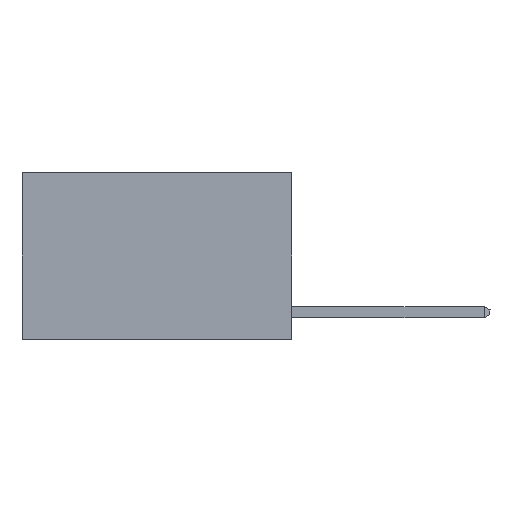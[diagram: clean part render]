
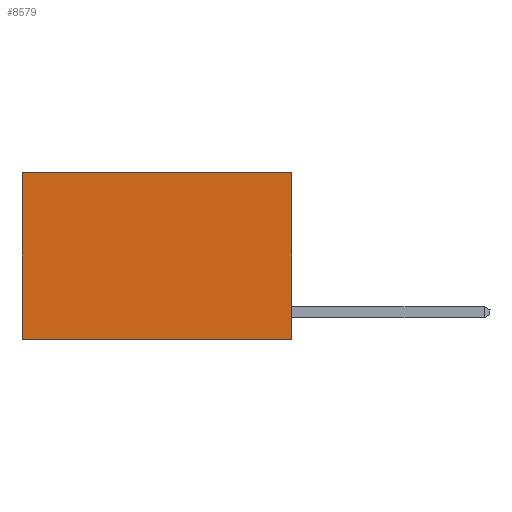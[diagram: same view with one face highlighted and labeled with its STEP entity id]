
A CAD part, left-side view. The second image highlights one B-rep face of the part: STEP entity #8579.
In plain terms, the highlighted planar face has unit normal (-1, 0, 0).
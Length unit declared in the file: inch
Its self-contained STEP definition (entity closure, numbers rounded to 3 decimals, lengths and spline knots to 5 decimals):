
#87 = DIRECTION ( 'NONE',  ( 0., 0., -1. ) ) ;
#495 = CARTESIAN_POINT ( 'NONE',  ( 0.2625, 0., 0. ) ) ;
#580 = VERTEX_POINT ( 'NONE', #14620 ) ;
#915 = VECTOR ( 'NONE', #23590, 39.37008 ) ;
#3266 = ORIENTED_EDGE ( 'NONE', *, *, #17826, .T. ) ;
#4470 = VECTOR ( 'NONE', #14200, 39.37008 ) ;
#4863 = LINE ( 'NONE', #22517, #13359 ) ;
#6535 = CARTESIAN_POINT ( 'NONE',  ( 0.2625, 0.6, -0.37 ) ) ;
#6614 = CARTESIAN_POINT ( 'NONE',  ( 0.2625, 0., 0. ) ) ;
#6972 = ORIENTED_EDGE ( 'NONE', *, *, #18097, .F. ) ;
#7374 = DIRECTION ( 'NONE',  ( 1., 0., 0. ) ) ;
#7459 = LINE ( 'NONE', #6614, #10046 ) ;
#8405 = EDGE_CURVE ( 'NONE', #580, #22793, #13631, .T. ) ;
#8579 = ADVANCED_FACE ( 'NONE', ( #9653 ), #20344, .F. ) ;
#9022 = CARTESIAN_POINT ( 'NONE',  ( 0.2625, 0.6, 0. ) ) ;
#9525 = EDGE_LOOP ( 'NONE', ( #20659, #10843, #6972, #3266 ) ) ;
#9653 = FACE_OUTER_BOUND ( 'NONE', #9525, .T. ) ;
#10037 = CARTESIAN_POINT ( 'NONE',  ( 0.2625, 0., -0.37 ) ) ;
#10046 = VECTOR ( 'NONE', #87, 39.37008 ) ;
#10719 = LINE ( 'NONE', #25592, #915 ) ;
#10843 = ORIENTED_EDGE ( 'NONE', *, *, #8405, .F. ) ;
#11716 = DIRECTION ( 'NONE',  ( 0., 0., -1. ) ) ;
#12298 = AXIS2_PLACEMENT_3D ( 'NONE', #26282, #7374, #11716 ) ;
#13359 = VECTOR ( 'NONE', #24653, 39.37008 ) ;
#13631 = LINE ( 'NONE', #10037, #4470 ) ;
#14200 = DIRECTION ( 'NONE',  ( 0., 1., 0. ) ) ;
#14620 = CARTESIAN_POINT ( 'NONE',  ( 0.2625, 0., -0.37 ) ) ;
#17826 = EDGE_CURVE ( 'NONE', #25338, #27219, #4863, .T. ) ;
#18097 = EDGE_CURVE ( 'NONE', #25338, #580, #7459, .T. ) ;
#20344 = PLANE ( 'NONE',  #12298 ) ;
#20659 = ORIENTED_EDGE ( 'NONE', *, *, #23370, .T. ) ;
#22517 = CARTESIAN_POINT ( 'NONE',  ( 0.2625, 0., 0. ) ) ;
#22793 = VERTEX_POINT ( 'NONE', #6535 ) ;
#23370 = EDGE_CURVE ( 'NONE', #27219, #22793, #10719, .T. ) ;
#23590 = DIRECTION ( 'NONE',  ( 0., 0., -1. ) ) ;
#24653 = DIRECTION ( 'NONE',  ( 0., 1., 0. ) ) ;
#25338 = VERTEX_POINT ( 'NONE', #495 ) ;
#25592 = CARTESIAN_POINT ( 'NONE',  ( 0.2625, 0.6, 0. ) ) ;
#26282 = CARTESIAN_POINT ( 'NONE',  ( 0.2625, 0., 0. ) ) ;
#27219 = VERTEX_POINT ( 'NONE', #9022 ) ;
